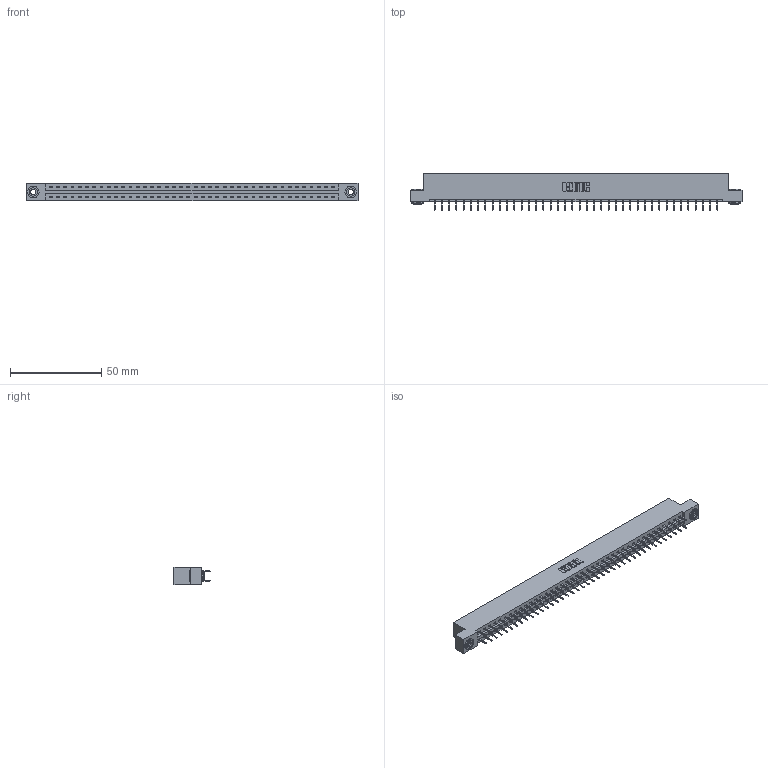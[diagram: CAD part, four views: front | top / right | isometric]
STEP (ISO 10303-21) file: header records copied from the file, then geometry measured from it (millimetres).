
FILE_DESCRIPTION (( 'STEP AP203' ), '1' );
FILE_NAME ('387-080-524-203.STEP', '2018-09-23T18:20:03', ( '' ), ( '' ), 'SwSTEP 2.0', 'SolidWorks 2016', '' );
FILE_SCHEMA (( 'CONFIG_CONTROL_DESIGN' ));
Length unit declared in the file: inch
Products named in the file (4): 345-250-002_345-250-002-102; 387-080-524-203; 337 Part_Flush Mounting Lugs - 0.156 Dia-TH; 345-292-001_345-293-124
Assembly tree (83 placements, depth 2):
  387-080-524-203
    337 Part_Flush Mounting Lugs - 0.156 Dia-TH
    345-292-001_345-293-124  x80
    345-250-002_345-250-002-102  x2
Bounding box: 181.51 x 19.69 x 9.4 mm (x, y, z)
Volume: 19000.5 mm3; surface area: 21310.1 mm2
Topology: 83 solids, 83 shells, 4792 faces, 13587 edges, 8734 vertices
Faces by surface type: plane 3600, cylinder 1184, cone 8
Entity records: 31996 total; most frequent: CARTESIAN_POINT 5365, ORIENTED_EDGE 5294, DIRECTION 4601, EDGE_CURVE 2647, VECTOR 2499, LINE 2499, VERTEX_POINT 1758, AXIS2_PLACEMENT_3D 1051
